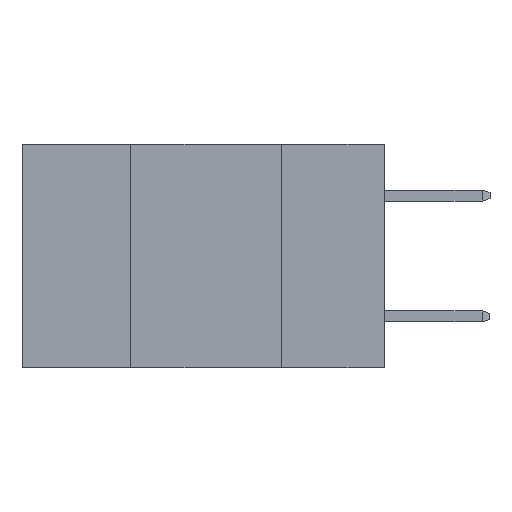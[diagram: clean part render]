
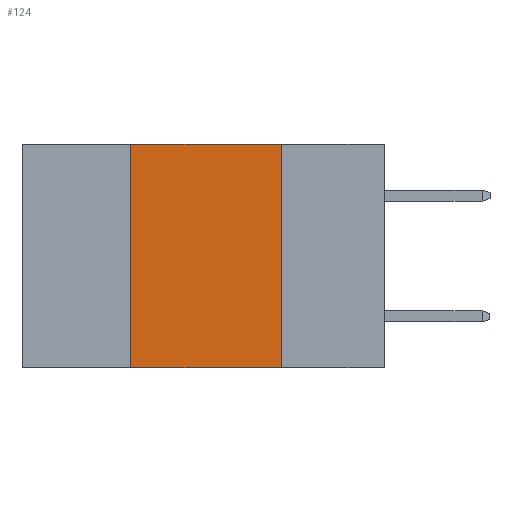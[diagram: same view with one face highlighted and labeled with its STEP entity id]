
A CAD part, left-side view. The second image highlights one B-rep face of the part: STEP entity #124.
In plain terms, the highlighted planar face has unit normal (-1, 0, 0).
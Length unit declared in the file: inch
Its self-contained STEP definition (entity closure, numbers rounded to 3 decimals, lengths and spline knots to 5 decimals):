
#19 = CARTESIAN_POINT ( 'NONE',  ( 0., 0.17, 0. ) ) ;
#124 = ADVANCED_FACE ( 'NONE', ( #1401 ), #9193, .F. ) ;
#1238 = DIRECTION ( 'NONE',  ( 0., 0., 1. ) ) ;
#1401 = FACE_OUTER_BOUND ( 'NONE', #11891, .T. ) ;
#1544 = VERTEX_POINT ( 'NONE', #5387 ) ;
#1988 = CARTESIAN_POINT ( 'NONE',  ( 0., 0.42, 0. ) ) ;
#2579 = ORIENTED_EDGE ( 'NONE', *, *, #3992, .F. ) ;
#2815 = CARTESIAN_POINT ( 'NONE',  ( 0., 0.17, 0. ) ) ;
#2978 = CARTESIAN_POINT ( 'NONE',  ( 0., 0.42, -0.37 ) ) ;
#3200 = VERTEX_POINT ( 'NONE', #2815 ) ;
#3343 = DIRECTION ( 'NONE',  ( 0., 0., -1. ) ) ;
#3992 = EDGE_CURVE ( 'NONE', #6938, #3200, #10000, .T. ) ;
#5113 = AXIS2_PLACEMENT_3D ( 'NONE', #9264, #5382, #3343 ) ;
#5226 = ORIENTED_EDGE ( 'NONE', *, *, #7173, .T. ) ;
#5382 = DIRECTION ( 'NONE',  ( 1., 0., 0. ) ) ;
#5387 = CARTESIAN_POINT ( 'NONE',  ( 0., 0.17, -0.37 ) ) ;
#6030 = VECTOR ( 'NONE', #18171, 39.37008 ) ;
#6481 = VECTOR ( 'NONE', #7797, 39.37008 ) ;
#6938 = VERTEX_POINT ( 'NONE', #10341 ) ;
#7173 = EDGE_CURVE ( 'NONE', #8122, #1544, #14284, .T. ) ;
#7797 = DIRECTION ( 'NONE',  ( 0., -1., 0. ) ) ;
#7839 = LINE ( 'NONE', #19, #18896 ) ;
#8054 = CARTESIAN_POINT ( 'NONE',  ( 0., 0.6, -0.37 ) ) ;
#8122 = VERTEX_POINT ( 'NONE', #2978 ) ;
#8167 = EDGE_CURVE ( 'NONE', #8122, #6938, #16956, .T. ) ;
#9170 = EDGE_CURVE ( 'NONE', #3200, #1544, #7839, .T. ) ;
#9193 = PLANE ( 'NONE',  #5113 ) ;
#9264 = CARTESIAN_POINT ( 'NONE',  ( 0., 0.6, 0. ) ) ;
#9284 = VECTOR ( 'NONE', #1238, 39.37008 ) ;
#10000 = LINE ( 'NONE', #12246, #6030 ) ;
#10341 = CARTESIAN_POINT ( 'NONE',  ( 0., 0.42, 0. ) ) ;
#10566 = ORIENTED_EDGE ( 'NONE', *, *, #9170, .F. ) ;
#11036 = ORIENTED_EDGE ( 'NONE', *, *, #8167, .F. ) ;
#11891 = EDGE_LOOP ( 'NONE', ( #10566, #2579, #11036, #5226 ) ) ;
#12246 = CARTESIAN_POINT ( 'NONE',  ( 0., 0.6, 0. ) ) ;
#14284 = LINE ( 'NONE', #8054, #6481 ) ;
#16415 = DIRECTION ( 'NONE',  ( 0., 0., -1. ) ) ;
#16956 = LINE ( 'NONE', #1988, #9284 ) ;
#18171 = DIRECTION ( 'NONE',  ( 0., -1., 0. ) ) ;
#18896 = VECTOR ( 'NONE', #16415, 39.37008 ) ;
